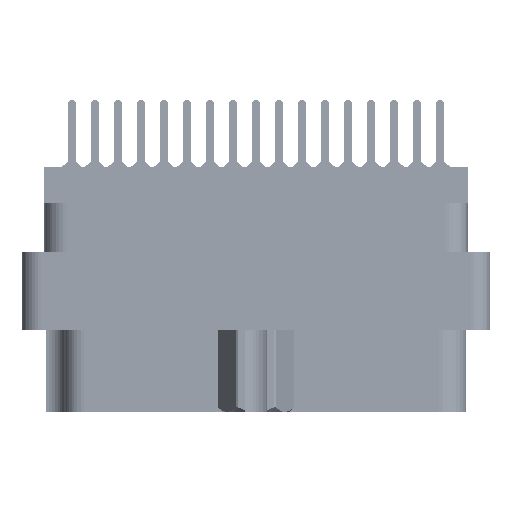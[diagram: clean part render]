
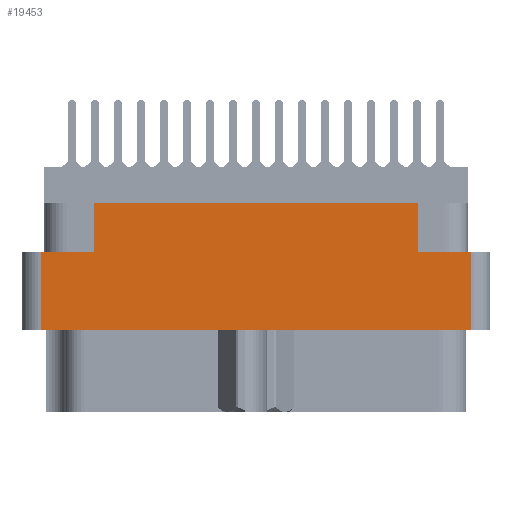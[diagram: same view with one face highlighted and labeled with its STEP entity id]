
A CAD part, left-side view. The second image highlights one B-rep face of the part: STEP entity #19453.
In plain terms, the highlighted planar face has unit normal (-1, 0, 0).
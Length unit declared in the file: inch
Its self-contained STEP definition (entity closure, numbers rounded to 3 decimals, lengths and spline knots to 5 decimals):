
#3002 = VECTOR ( 'NONE', #11012, 39.37008 ) ;
#6283 = LINE ( 'NONE', #51692, #18900 ) ;
#7329 = EDGE_CURVE ( 'NONE', #62009, #76667, #58277, .T. ) ;
#8030 = CARTESIAN_POINT ( 'NONE',  ( -1.375, -0.7005, -0.798 ) ) ;
#10488 = ORIENTED_EDGE ( 'NONE', *, *, #11205, .T. ) ;
#10862 = LINE ( 'NONE', #8030, #53396 ) ;
#11012 = DIRECTION ( 'NONE',  ( 0., -1., 0. ) ) ;
#11205 = EDGE_CURVE ( 'NONE', #55121, #27778, #10862, .T. ) ;
#11751 = VECTOR ( 'NONE', #81143, 39.37008 ) ;
#12107 = ORIENTED_EDGE ( 'NONE', *, *, #32299, .F. ) ;
#12898 = CARTESIAN_POINT ( 'NONE',  ( -1.375, 0.5285, -0.277 ) ) ;
#14530 = LINE ( 'NONE', #96761, #97105 ) ;
#15074 = EDGE_CURVE ( 'NONE', #55121, #76667, #79141, .T. ) ;
#16859 = EDGE_LOOP ( 'NONE', ( #72304, #89883, #101292, #10488, #44747, #69972, #12107, #55494 ) ) ;
#18900 = VECTOR ( 'NONE', #83191, 39.37008 ) ;
#19453 = ADVANCED_FACE ( 'NONE', ( #102807 ), #52898, .T. ) ;
#26249 = CARTESIAN_POINT ( 'NONE',  ( -1.375, 0.7625, -0.117 ) ) ;
#26852 = LINE ( 'NONE', #26249, #11751 ) ;
#27778 = VERTEX_POINT ( 'NONE', #79195 ) ;
#30284 = VECTOR ( 'NONE', #85273, 39.37008 ) ;
#30405 = EDGE_CURVE ( 'NONE', #36652, #27778, #85604, .T. ) ;
#32299 = EDGE_CURVE ( 'NONE', #48013, #88507, #26852, .T. ) ;
#36652 = VERTEX_POINT ( 'NONE', #59850 ) ;
#38615 = EDGE_CURVE ( 'NONE', #36652, #88507, #6283, .T. ) ;
#41696 = CARTESIAN_POINT ( 'NONE',  ( -1.375, -0.7005, -0.529 ) ) ;
#44747 = ORIENTED_EDGE ( 'NONE', *, *, #30405, .F. ) ;
#47471 = AXIS2_PLACEMENT_3D ( 'NONE', #101873, #78089, #77764 ) ;
#48013 = VERTEX_POINT ( 'NONE', #67045 ) ;
#50340 = DIRECTION ( 'NONE',  ( 0., 0., -1. ) ) ;
#51559 = LINE ( 'NONE', #12898, #30284 ) ;
#51689 = CARTESIAN_POINT ( 'NONE',  ( -1.375, -0.5285, -0.117 ) ) ;
#51692 = CARTESIAN_POINT ( 'NONE',  ( -1.375, -0.5285, -0.277 ) ) ;
#52898 = PLANE ( 'NONE',  #47471 ) ;
#53396 = VECTOR ( 'NONE', #65000, 39.37008 ) ;
#55121 = VERTEX_POINT ( 'NONE', #41696 ) ;
#55494 = ORIENTED_EDGE ( 'NONE', *, *, #66756, .F. ) ;
#57905 = CARTESIAN_POINT ( 'NONE',  ( -1.375, 0.5285, -0.277 ) ) ;
#58277 = LINE ( 'NONE', #90603, #83260 ) ;
#58676 = CARTESIAN_POINT ( 'NONE',  ( -1.375, 0.7005, -0.529 ) ) ;
#59850 = CARTESIAN_POINT ( 'NONE',  ( -1.375, -0.5285, -0.277 ) ) ;
#62009 = VERTEX_POINT ( 'NONE', #99536 ) ;
#65000 = DIRECTION ( 'NONE',  ( 0., 0., 1. ) ) ;
#66756 = EDGE_CURVE ( 'NONE', #68319, #48013, #51559, .T. ) ;
#67045 = CARTESIAN_POINT ( 'NONE',  ( -1.375, 0.5285, -0.117 ) ) ;
#68319 = VERTEX_POINT ( 'NONE', #57905 ) ;
#69972 = ORIENTED_EDGE ( 'NONE', *, *, #38615, .T. ) ;
#71896 = DIRECTION ( 'NONE',  ( 0., 1., 0. ) ) ;
#72304 = ORIENTED_EDGE ( 'NONE', *, *, #88940, .F. ) ;
#76667 = VERTEX_POINT ( 'NONE', #58676 ) ;
#77764 = DIRECTION ( 'NONE',  ( 0., 0., 1. ) ) ;
#78089 = DIRECTION ( 'NONE',  ( -1., 0., 0. ) ) ;
#79141 = LINE ( 'NONE', #100701, #96622 ) ;
#79195 = CARTESIAN_POINT ( 'NONE',  ( -1.375, -0.7005, -0.277 ) ) ;
#81143 = DIRECTION ( 'NONE',  ( 0., -1., 0. ) ) ;
#83191 = DIRECTION ( 'NONE',  ( 0., 0., 1. ) ) ;
#83260 = VECTOR ( 'NONE', #50340, 39.37008 ) ;
#83421 = CARTESIAN_POINT ( 'NONE',  ( -1.375, 0., -0.277 ) ) ;
#85273 = DIRECTION ( 'NONE',  ( 0., 0., 1. ) ) ;
#85604 = LINE ( 'NONE', #83421, #3002 ) ;
#88507 = VERTEX_POINT ( 'NONE', #51689 ) ;
#88940 = EDGE_CURVE ( 'NONE', #62009, #68319, #14530, .T. ) ;
#89883 = ORIENTED_EDGE ( 'NONE', *, *, #7329, .T. ) ;
#90603 = CARTESIAN_POINT ( 'NONE',  ( -1.375, 0.7005, -0.798 ) ) ;
#96622 = VECTOR ( 'NONE', #71896, 39.37008 ) ;
#96761 = CARTESIAN_POINT ( 'NONE',  ( -1.375, 0., -0.277 ) ) ;
#97105 = VECTOR ( 'NONE', #97820, 39.37008 ) ;
#97820 = DIRECTION ( 'NONE',  ( 0., -1., 0. ) ) ;
#99536 = CARTESIAN_POINT ( 'NONE',  ( -1.375, 0.7005, -0.277 ) ) ;
#100701 = CARTESIAN_POINT ( 'NONE',  ( -1.375, 0., -0.529 ) ) ;
#101292 = ORIENTED_EDGE ( 'NONE', *, *, #15074, .F. ) ;
#101873 = CARTESIAN_POINT ( 'NONE',  ( -1.375, -0.7625, -0.798 ) ) ;
#102807 = FACE_OUTER_BOUND ( 'NONE', #16859, .T. ) ;
